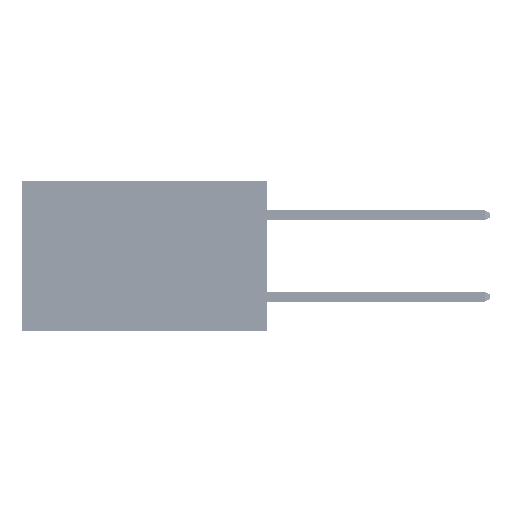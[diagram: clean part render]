
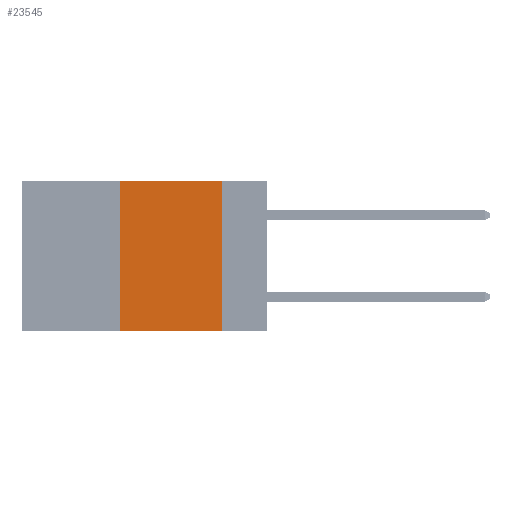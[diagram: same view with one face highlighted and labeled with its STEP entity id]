
A CAD part, left-side view. The second image highlights one B-rep face of the part: STEP entity #23545.
In plain terms, the highlighted planar face has unit normal (-1, 0, 0).
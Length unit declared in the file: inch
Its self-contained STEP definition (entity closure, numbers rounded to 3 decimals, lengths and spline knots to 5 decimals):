
#95 = ORIENTED_EDGE ( 'NONE', *, *, #24631, .F. ) ;
#6032 = EDGE_CURVE ( 'NONE', #49344, #44847, #11758, .T. ) ;
#11758 = LINE ( 'NONE', #51784, #42389 ) ;
#12898 = VERTEX_POINT ( 'NONE', #48291 ) ;
#16009 = CARTESIAN_POINT ( 'NONE',  ( 0., 0.11, 0. ) ) ;
#16663 = AXIS2_PLACEMENT_3D ( 'NONE', #48302, #36212, #23955 ) ;
#17456 = VECTOR ( 'NONE', #45745, 39.37008 ) ;
#20094 = PLANE ( 'NONE',  #16663 ) ;
#20773 = CARTESIAN_POINT ( 'NONE',  ( 0., 0.11, -0.37 ) ) ;
#22700 = ORIENTED_EDGE ( 'NONE', *, *, #37519, .F. ) ;
#23545 = ADVANCED_FACE ( 'NONE', ( #37562 ), #20094, .F. ) ;
#23955 = DIRECTION ( 'NONE',  ( 0., 0., -1. ) ) ;
#24242 = VERTEX_POINT ( 'NONE', #20773 ) ;
#24631 = EDGE_CURVE ( 'NONE', #44847, #12898, #43737, .T. ) ;
#24782 = ORIENTED_EDGE ( 'NONE', *, *, #26881, .T. ) ;
#26881 = EDGE_CURVE ( 'NONE', #49344, #24242, #43819, .T. ) ;
#27568 = VECTOR ( 'NONE', #30866, 39.37008 ) ;
#30866 = DIRECTION ( 'NONE',  ( 0., -1., 0. ) ) ;
#31709 = VECTOR ( 'NONE', #48039, 39.37008 ) ;
#31783 = CARTESIAN_POINT ( 'NONE',  ( 0., 0.36, -0.37 ) ) ;
#33521 = ORIENTED_EDGE ( 'NONE', *, *, #6032, .F. ) ;
#35280 = DIRECTION ( 'NONE',  ( 0., 0., 1. ) ) ;
#35281 = CARTESIAN_POINT ( 'NONE',  ( 0., 0.36, 0. ) ) ;
#36212 = DIRECTION ( 'NONE',  ( 1., 0., 0. ) ) ;
#37376 = CARTESIAN_POINT ( 'NONE',  ( 0., 0.6, 0. ) ) ;
#37519 = EDGE_CURVE ( 'NONE', #12898, #24242, #43621, .T. ) ;
#37562 = FACE_OUTER_BOUND ( 'NONE', #51276, .T. ) ;
#42389 = VECTOR ( 'NONE', #35280, 39.37008 ) ;
#42588 = CARTESIAN_POINT ( 'NONE',  ( 0., 0.6, -0.37 ) ) ;
#43621 = LINE ( 'NONE', #16009, #31709 ) ;
#43737 = LINE ( 'NONE', #37376, #17456 ) ;
#43819 = LINE ( 'NONE', #42588, #27568 ) ;
#44847 = VERTEX_POINT ( 'NONE', #35281 ) ;
#45745 = DIRECTION ( 'NONE',  ( 0., -1., 0. ) ) ;
#48039 = DIRECTION ( 'NONE',  ( 0., 0., -1. ) ) ;
#48291 = CARTESIAN_POINT ( 'NONE',  ( 0., 0.11, 0. ) ) ;
#48302 = CARTESIAN_POINT ( 'NONE',  ( 0., 0.6, 0. ) ) ;
#49344 = VERTEX_POINT ( 'NONE', #31783 ) ;
#51276 = EDGE_LOOP ( 'NONE', ( #22700, #95, #33521, #24782 ) ) ;
#51784 = CARTESIAN_POINT ( 'NONE',  ( 0., 0.36, 0. ) ) ;
